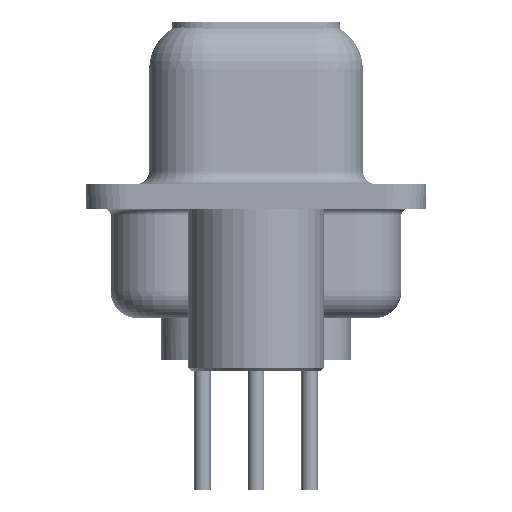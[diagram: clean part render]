
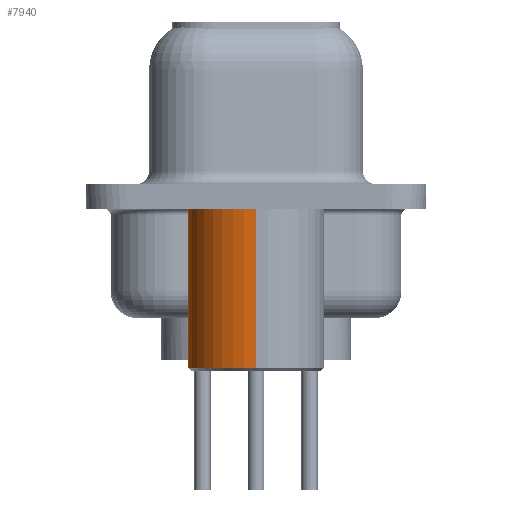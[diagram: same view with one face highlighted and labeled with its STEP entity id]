
A CAD part, left-side view. The second image highlights one B-rep face of the part: STEP entity #7940.
In plain terms, the highlighted cylindrical face has radius 2.5 mm (diameter 5 mm), a partial arc.
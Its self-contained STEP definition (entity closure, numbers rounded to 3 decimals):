
#848 = CIRCLE ( 'NONE', #6060, 2.5 ) ;
#971 = EDGE_CURVE ( 'NONE', #23373, #20318, #848, .T. ) ;
#2095 = DIRECTION ( 'NONE',  ( 0., 0., 1. ) ) ;
#2781 = DIRECTION ( 'NONE',  ( 0., 0., 1. ) ) ;
#5118 = EDGE_CURVE ( 'NONE', #11035, #23373, #27913, .T. ) ;
#5254 = CARTESIAN_POINT ( 'NONE',  ( 0., 0., -0.45 ) ) ;
#5889 = AXIS2_PLACEMENT_3D ( 'NONE', #16312, #37638, #18765 ) ;
#5895 = AXIS2_PLACEMENT_3D ( 'NONE', #36646, #2781, #14703 ) ;
#6060 = AXIS2_PLACEMENT_3D ( 'NONE', #5254, #17780, #15086 ) ;
#7857 = EDGE_LOOP ( 'NONE', ( #15278, #11563, #18280, #25444 ) ) ;
#7940 = ADVANCED_FACE ( 'NONE', ( #24161 ), #27448, .T. ) ;
#8874 = VECTOR ( 'NONE', #2095, 1000. ) ;
#11035 = VERTEX_POINT ( 'NONE', #19101 ) ;
#11563 = ORIENTED_EDGE ( 'NONE', *, *, #17805, .T. ) ;
#14703 = DIRECTION ( 'NONE',  ( 1., 0., 0. ) ) ;
#15086 = DIRECTION ( 'NONE',  ( 1., 0., 0. ) ) ;
#15278 = ORIENTED_EDGE ( 'NONE', *, *, #25675, .T. ) ;
#15583 = CARTESIAN_POINT ( 'NONE',  ( 2.5, 0., 0.581 ) ) ;
#16312 = CARTESIAN_POINT ( 'NONE',  ( 0., 0., -6.35 ) ) ;
#17780 = DIRECTION ( 'NONE',  ( 0., 0., 1. ) ) ;
#17805 = EDGE_CURVE ( 'NONE', #31775, #20318, #35950, .T. ) ;
#18280 = ORIENTED_EDGE ( 'NONE', *, *, #971, .F. ) ;
#18765 = DIRECTION ( 'NONE',  ( 1., 0., 0. ) ) ;
#19101 = CARTESIAN_POINT ( 'NONE',  ( 2.5, 0., -6.35 ) ) ;
#20229 = CARTESIAN_POINT ( 'NONE',  ( -2.5, 0., -0.45 ) ) ;
#20318 = VERTEX_POINT ( 'NONE', #20229 ) ;
#22980 = CIRCLE ( 'NONE', #5889, 2.5 ) ;
#23373 = VERTEX_POINT ( 'NONE', #25671 ) ;
#24161 = FACE_OUTER_BOUND ( 'NONE', #7857, .T. ) ;
#25444 = ORIENTED_EDGE ( 'NONE', *, *, #5118, .F. ) ;
#25671 = CARTESIAN_POINT ( 'NONE',  ( 2.5, 0., -0.45 ) ) ;
#25675 = EDGE_CURVE ( 'NONE', #11035, #31775, #22980, .T. ) ;
#27448 = CYLINDRICAL_SURFACE ( 'NONE', #5895, 2.5 ) ;
#27913 = LINE ( 'NONE', #15583, #28831 ) ;
#28831 = VECTOR ( 'NONE', #30774, 1000. ) ;
#28951 = CARTESIAN_POINT ( 'NONE',  ( -2.5, 0., -6.35 ) ) ;
#30774 = DIRECTION ( 'NONE',  ( 0., 0., 1. ) ) ;
#31775 = VERTEX_POINT ( 'NONE', #28951 ) ;
#35950 = LINE ( 'NONE', #38860, #8874 ) ;
#36646 = CARTESIAN_POINT ( 'NONE',  ( 0., 0., 0.581 ) ) ;
#37638 = DIRECTION ( 'NONE',  ( 0., 0., 1. ) ) ;
#38860 = CARTESIAN_POINT ( 'NONE',  ( -2.5, 0., 0.581 ) ) ;
